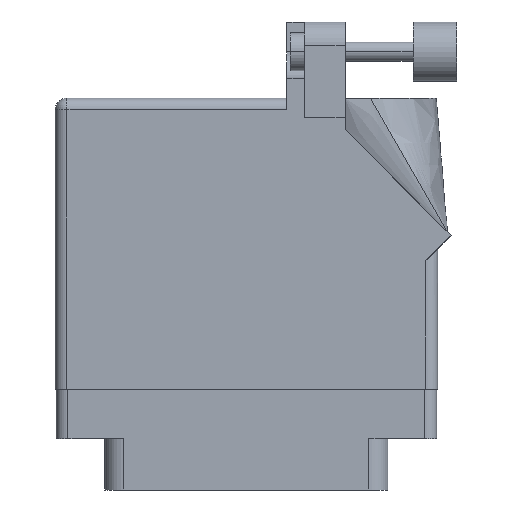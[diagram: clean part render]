
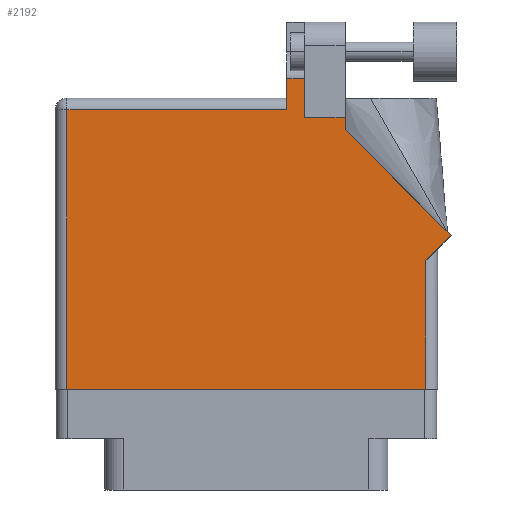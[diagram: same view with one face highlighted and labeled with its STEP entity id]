
A CAD part, front view. The second image highlights one B-rep face of the part: STEP entity #2192.
In plain terms, the highlighted face is planar.
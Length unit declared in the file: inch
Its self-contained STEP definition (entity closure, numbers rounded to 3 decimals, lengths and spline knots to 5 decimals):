
#573 = DIRECTION ( 'NONE',  ( -1., 0., 0. ) ) ;
#696 = EDGE_CURVE ( 'NONE', #5420, #30097, #38115, .T. ) ;
#729 = VECTOR ( 'NONE', #23781, 39.37008 ) ;
#765 = CARTESIAN_POINT ( 'NONE',  ( 0., 1.468, 0. ) ) ;
#2192 = ADVANCED_FACE ( 'NONE', ( #38791 ), #12319, .F. ) ;
#2265 = LINE ( 'NONE', #11008, #18397 ) ;
#2302 = EDGE_CURVE ( 'NONE', #30097, #34008, #3958, .T. ) ;
#2354 = EDGE_CURVE ( 'NONE', #34008, #36602, #19053, .T. ) ;
#2927 = VERTEX_POINT ( 'NONE', #25560 ) ;
#3340 = VECTOR ( 'NONE', #30832, 39.37008 ) ;
#3958 = LINE ( 'NONE', #33810, #3340 ) ;
#5329 = ORIENTED_EDGE ( 'NONE', *, *, #2302, .T. ) ;
#5420 = VERTEX_POINT ( 'NONE', #18483 ) ;
#6061 = ORIENTED_EDGE ( 'NONE', *, *, #32596, .T. ) ;
#6238 = CARTESIAN_POINT ( 'NONE',  ( 0., 0., 0. ) ) ;
#6315 = VECTOR ( 'NONE', #10390, 39.37008 ) ;
#9345 = DIRECTION ( 'NONE',  ( 0., 0., -1. ) ) ;
#10390 = DIRECTION ( 'NONE',  ( -1., 0., 0. ) ) ;
#10844 = DIRECTION ( 'NONE',  ( -1., 0., 0. ) ) ;
#11008 = CARTESIAN_POINT ( 'NONE',  ( 2.08071, 0.80771, 0. ) ) ;
#11202 = DIRECTION ( 'NONE',  ( -0.707, 0.707, 0. ) ) ;
#11524 = VECTOR ( 'NONE', #14237, 39.37008 ) ;
#11749 = DIRECTION ( 'NONE',  ( 0.707, 0.707, 0. ) ) ;
#11802 = LINE ( 'NONE', #6238, #35746 ) ;
#12257 = CARTESIAN_POINT ( 'NONE',  ( 1.524, 1.36442, 0. ) ) ;
#12319 = PLANE ( 'NONE',  #22983 ) ;
#12660 = ORIENTED_EDGE ( 'NONE', *, *, #28553, .T. ) ;
#14167 = VECTOR ( 'NONE', #23585, 39.37008 ) ;
#14237 = DIRECTION ( 'NONE',  ( 0., 1., 0. ) ) ;
#14990 = CARTESIAN_POINT ( 'NONE',  ( 1.217, 1.468, 0. ) ) ;
#15120 = CARTESIAN_POINT ( 'NONE',  ( 2.01, 0.737, 0. ) ) ;
#15455 = VERTEX_POINT ( 'NONE', #12257 ) ;
#15679 = CARTESIAN_POINT ( 'NONE',  ( 1.311, 1.43, 0. ) ) ;
#15954 = CARTESIAN_POINT ( 'NONE',  ( 1.524, 1.43, 0. ) ) ;
#16232 = VERTEX_POINT ( 'NONE', #15679 ) ;
#17274 = CARTESIAN_POINT ( 'NONE',  ( 1.217, 1.6315, 0. ) ) ;
#17670 = ORIENTED_EDGE ( 'NONE', *, *, #696, .T. ) ;
#17808 = CARTESIAN_POINT ( 'NONE',  ( 1.524, 1.36442, 0. ) ) ;
#18011 = LINE ( 'NONE', #27343, #729 ) ;
#18397 = VECTOR ( 'NONE', #11202, 39.37008 ) ;
#18483 = CARTESIAN_POINT ( 'NONE',  ( 1.311, 1.6315, 0. ) ) ;
#19053 = LINE ( 'NONE', #765, #34462 ) ;
#20989 = CARTESIAN_POINT ( 'NONE',  ( 0.062, 0., 0. ) ) ;
#21185 = EDGE_CURVE ( 'NONE', #36014, #15455, #2265, .T. ) ;
#21554 = VERTEX_POINT ( 'NONE', #28076 ) ;
#21675 = VECTOR ( 'NONE', #10844, 39.37008 ) ;
#22983 = AXIS2_PLACEMENT_3D ( 'NONE', #30037, #9345, #36202 ) ;
#23378 = CARTESIAN_POINT ( 'NONE',  ( 1.64177, 1.6315, 0. ) ) ;
#23585 = DIRECTION ( 'NONE',  ( 0., -1., 0. ) ) ;
#23781 = DIRECTION ( 'NONE',  ( 0., 1., 0. ) ) ;
#24056 = ORIENTED_EDGE ( 'NONE', *, *, #25268, .T. ) ;
#25248 = EDGE_LOOP ( 'NONE', ( #26738, #17670, #5329, #33235, #35087, #6061, #24056, #12660, #36947, #31805, #26837 ) ) ;
#25268 = EDGE_CURVE ( 'NONE', #21554, #29997, #18011, .T. ) ;
#25560 = CARTESIAN_POINT ( 'NONE',  ( 1.524, 1.43, 0. ) ) ;
#26432 = VERTEX_POINT ( 'NONE', #28086 ) ;
#26738 = ORIENTED_EDGE ( 'NONE', *, *, #27124, .T. ) ;
#26758 = LINE ( 'NONE', #20989, #14167 ) ;
#26837 = ORIENTED_EDGE ( 'NONE', *, *, #37452, .T. ) ;
#27124 = EDGE_CURVE ( 'NONE', #16232, #5420, #31357, .T. ) ;
#27343 = CARTESIAN_POINT ( 'NONE',  ( 1.948, 0.737, 0. ) ) ;
#28076 = CARTESIAN_POINT ( 'NONE',  ( 1.948, 0., 0. ) ) ;
#28086 = CARTESIAN_POINT ( 'NONE',  ( 0.062, 0., 0. ) ) ;
#28553 = EDGE_CURVE ( 'NONE', #29997, #36014, #33256, .T. ) ;
#29101 = VECTOR ( 'NONE', #11749, 39.37008 ) ;
#29997 = VERTEX_POINT ( 'NONE', #31446 ) ;
#30037 = CARTESIAN_POINT ( 'NONE',  ( 0., 1.53, 0. ) ) ;
#30097 = VERTEX_POINT ( 'NONE', #17274 ) ;
#30832 = DIRECTION ( 'NONE',  ( 0., -1., 0. ) ) ;
#31357 = LINE ( 'NONE', #32690, #34877 ) ;
#31446 = CARTESIAN_POINT ( 'NONE',  ( 1.948, 0.675, 0. ) ) ;
#31805 = ORIENTED_EDGE ( 'NONE', *, *, #32010, .T. ) ;
#32010 = EDGE_CURVE ( 'NONE', #15455, #2927, #32365, .T. ) ;
#32127 = CARTESIAN_POINT ( 'NONE',  ( 2.08071, 0.80771, 0. ) ) ;
#32365 = LINE ( 'NONE', #17808, #11524 ) ;
#32596 = EDGE_CURVE ( 'NONE', #26432, #21554, #11802, .T. ) ;
#32690 = CARTESIAN_POINT ( 'NONE',  ( 1.311, 1.43, 0. ) ) ;
#33235 = ORIENTED_EDGE ( 'NONE', *, *, #2354, .T. ) ;
#33256 = LINE ( 'NONE', #15120, #29101 ) ;
#33395 = EDGE_CURVE ( 'NONE', #36602, #26432, #26758, .T. ) ;
#33810 = CARTESIAN_POINT ( 'NONE',  ( 1.217, 1.53, 0. ) ) ;
#34008 = VERTEX_POINT ( 'NONE', #14990 ) ;
#34331 = DIRECTION ( 'NONE',  ( 0., 1., 0. ) ) ;
#34462 = VECTOR ( 'NONE', #573, 39.37008 ) ;
#34877 = VECTOR ( 'NONE', #34331, 39.37008 ) ;
#35087 = ORIENTED_EDGE ( 'NONE', *, *, #33395, .T. ) ;
#35746 = VECTOR ( 'NONE', #36273, 39.37008 ) ;
#36014 = VERTEX_POINT ( 'NONE', #32127 ) ;
#36202 = DIRECTION ( 'NONE',  ( -1., 0., 0. ) ) ;
#36273 = DIRECTION ( 'NONE',  ( 1., 0., 0. ) ) ;
#36602 = VERTEX_POINT ( 'NONE', #37599 ) ;
#36947 = ORIENTED_EDGE ( 'NONE', *, *, #21185, .T. ) ;
#37077 = LINE ( 'NONE', #15954, #6315 ) ;
#37452 = EDGE_CURVE ( 'NONE', #2927, #16232, #37077, .T. ) ;
#37599 = CARTESIAN_POINT ( 'NONE',  ( 0.062, 1.468, 0. ) ) ;
#38115 = LINE ( 'NONE', #23378, #21675 ) ;
#38791 = FACE_OUTER_BOUND ( 'NONE', #25248, .T. ) ;
